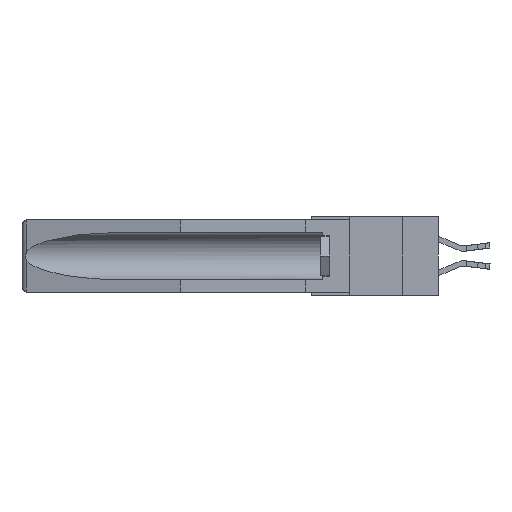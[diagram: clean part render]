
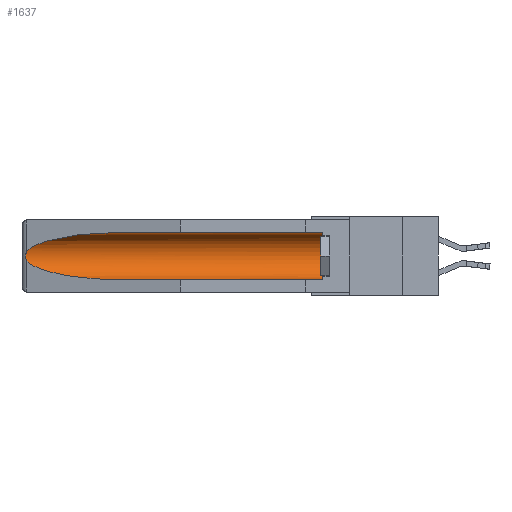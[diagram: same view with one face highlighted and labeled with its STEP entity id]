
A CAD part, left-side view. The second image highlights one B-rep face of the part: STEP entity #1637.
In plain terms, the highlighted cylindrical face has radius 2.857 mm (diameter 5.715 mm), a partial arc.
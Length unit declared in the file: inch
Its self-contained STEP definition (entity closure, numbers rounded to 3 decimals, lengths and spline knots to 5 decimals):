
#1419 = CARTESIAN_POINT ( 'NONE',  ( 0.2675, 1.53308, -0.17534 ) ) ;
#1426 = LINE ( 'NONE', #3609, #10726 ) ;
#1553 = CARTESIAN_POINT ( 'NONE',  ( 0.26537, 1.52718, -0.19328 ) ) ;
#1637 = ADVANCED_FACE ( 'NONE', ( #7533 ), #21561, .F. ) ;
#1683 = CARTESIAN_POINT ( 'NONE',  ( 0.21114, 1.30732, -0.059 ) ) ;
#1746 = EDGE_CURVE ( 'NONE', #3639, #2605, #24716, .T. ) ;
#2605 = VERTEX_POINT ( 'NONE', #8621 ) ;
#3057 = CARTESIAN_POINT ( 'NONE',  ( 0.155, -0.30754, -0.1715 ) ) ;
#3138 = DIRECTION ( 'NONE',  ( 0., 0., 1. ) ) ;
#3371 = CARTESIAN_POINT ( 'NONE',  ( 0.26537, 1.52718, -0.14972 ) ) ;
#3412 = CARTESIAN_POINT ( 'NONE',  ( 0.2673, 1.53269, -0.17917 ) ) ;
#3609 = CARTESIAN_POINT ( 'NONE',  ( 0.155, -0.30754, -0.284 ) ) ;
#3639 = VERTEX_POINT ( 'NONE', #21861 ) ;
#3645 = CARTESIAN_POINT ( 'NONE',  ( 0.155, 1.07973, -0.284 ) ) ;
#5535 = DIRECTION ( 'NONE',  ( 0., 1., 0. ) ) ;
#7226 = VERTEX_POINT ( 'NONE', #24868 ) ;
#7533 = FACE_OUTER_BOUND ( 'NONE', #17918, .T. ) ;
#7554 = DIRECTION ( 'NONE',  ( 0., 1., 0. ) ) ;
#7631 = CARTESIAN_POINT ( 'NONE',  ( 0.26537, 1.52718, -0.14972 ) ) ;
#7634 = EDGE_CURVE ( 'NONE', #20573, #3639, #15903, .T. ) ;
#8621 = CARTESIAN_POINT ( 'NONE',  ( 0.155, 1.07973, -0.059 ) ) ;
#9379 = EDGE_CURVE ( 'NONE', #22008, #7226, #23030, .T. ) ;
#9473 = ORIENTED_EDGE ( 'NONE', *, *, #21713, .T. ) ;
#9589 = CARTESIAN_POINT ( 'NONE',  ( 0.155, 0.126, -0.284 ) ) ;
#9754 = ORIENTED_EDGE ( 'NONE', *, *, #9379, .T. ) ;
#10726 = VECTOR ( 'NONE', #7554, 39.37008 ) ;
#11158 = ORIENTED_EDGE ( 'NONE', *, *, #1746, .T. ) ;
#11304 = CARTESIAN_POINT ( 'NONE',  ( 0.26654, 1.53092, -0.15636 ) ) ;
#11393 = VERTEX_POINT ( 'NONE', #3371 ) ;
#11518 = CARTESIAN_POINT ( 'NONE',  ( 0.155, -0.30754, -0.059 ) ) ;
#12399 = DIRECTION ( 'NONE',  ( 0., 0., 1. ) ) ;
#12753 = EDGE_CURVE ( 'NONE', #20573, #7226, #1426, .T. ) ;
#13455 = CARTESIAN_POINT ( 'NONE',  ( 0.2673, 1.5327, -0.16383 ) ) ;
#13699 = EDGE_CURVE ( 'NONE', #2605, #11393, #17578, .T. ) ;
#14165 = CARTESIAN_POINT ( 'NONE',  ( 0.26537, 1.52718, -0.19328 ) ) ;
#14241 = CARTESIAN_POINT ( 'NONE',  ( 0.155, 0.126, -0.1715 ) ) ;
#15210 = CARTESIAN_POINT ( 'NONE',  ( 0.155, 1.07973, -0.059 ) ) ;
#15285 = CARTESIAN_POINT ( 'NONE',  ( 0.26597, 1.52961, -0.15275 ) ) ;
#15370 = CARTESIAN_POINT ( 'NONE',  ( 0.26537, 1.52718, -0.14972 ) ) ;
#15903 = CIRCLE ( 'NONE', #24970, 0.1125 ) ;
#17293 = CARTESIAN_POINT ( 'NONE',  ( 0.26537, 1.52718, -0.19328 ) ) ;
#17344 = CARTESIAN_POINT ( 'NONE',  ( 0.21114, 1.30732, -0.284 ) ) ;
#17375 = CARTESIAN_POINT ( 'NONE',  ( 0.2675, 1.53308, -0.16763 ) ) ;
#17578 =( BOUNDED_CURVE ( )  B_SPLINE_CURVE ( 3, ( #15210, #1683, #23603, #7631 ),
 .UNSPECIFIED., .F., .T. ) 
 B_SPLINE_CURVE_WITH_KNOTS ( ( 4, 4 ),
 ( 4.71239, 6.08839 ),
 .UNSPECIFIED. ) 
 CURVE ( )  GEOMETRIC_REPRESENTATION_ITEM ( )  RATIONAL_B_SPLINE_CURVE ( ( 1., 0.848, 0.848, 1. ) ) 
 REPRESENTATION_ITEM ( '' )  );
#17918 = EDGE_LOOP ( 'NONE', ( #19096, #9473, #9754, #24249, #18163, #11158 ) ) ;
#18163 = ORIENTED_EDGE ( 'NONE', *, *, #7634, .T. ) ;
#19096 = ORIENTED_EDGE ( 'NONE', *, *, #13699, .T. ) ;
#19286 = CARTESIAN_POINT ( 'NONE',  ( 0.26655, 1.53094, -0.18657 ) ) ;
#19682 = VECTOR ( 'NONE', #5535, 39.37008 ) ;
#20573 = VERTEX_POINT ( 'NONE', #9589 ) ;
#20808 = B_SPLINE_CURVE_WITH_KNOTS ( 'NONE', 3,
 ( #15370, #15285, #11304, #13455, #17375, #1419, #3412, #19286, #21478, #17293 ),
 .UNSPECIFIED., .F., .F.,
 ( 4, 2, 2, 2, 4 ),
 ( 0., 0.00029, 0.00058, 0.00087, 0.00117 ),
 .UNSPECIFIED. ) ;
#21478 = CARTESIAN_POINT ( 'NONE',  ( 0.26597, 1.5296, -0.19026 ) ) ;
#21561 = CYLINDRICAL_SURFACE ( 'NONE', #23545, 0.1125 ) ;
#21713 = EDGE_CURVE ( 'NONE', #11393, #22008, #20808, .T. ) ;
#21861 = CARTESIAN_POINT ( 'NONE',  ( 0.155, 0.126, -0.059 ) ) ;
#22008 = VERTEX_POINT ( 'NONE', #14165 ) ;
#22167 = DIRECTION ( 'NONE',  ( 0., -1., 0. ) ) ;
#23030 =( BOUNDED_CURVE ( )  B_SPLINE_CURVE ( 3, ( #1553, #25505, #17344, #3645 ),
 .UNSPECIFIED., .F., .F. ) 
 B_SPLINE_CURVE_WITH_KNOTS ( ( 4, 4 ),
 ( 0.1948, 1.5708 ),
 .UNSPECIFIED. ) 
 CURVE ( )  GEOMETRIC_REPRESENTATION_ITEM ( )  RATIONAL_B_SPLINE_CURVE ( ( 1., 0.848, 0.848, 1. ) ) 
 REPRESENTATION_ITEM ( '' )  );
#23545 = AXIS2_PLACEMENT_3D ( 'NONE', #3057, #24976, #3138 ) ;
#23603 = CARTESIAN_POINT ( 'NONE',  ( 0.25451, 1.48313, -0.09465 ) ) ;
#24249 = ORIENTED_EDGE ( 'NONE', *, *, #12753, .F. ) ;
#24716 = LINE ( 'NONE', #11518, #19682 ) ;
#24868 = CARTESIAN_POINT ( 'NONE',  ( 0.155, 1.07973, -0.284 ) ) ;
#24970 = AXIS2_PLACEMENT_3D ( 'NONE', #14241, #22167, #12399 ) ;
#24976 = DIRECTION ( 'NONE',  ( 0., 1., 0. ) ) ;
#25505 = CARTESIAN_POINT ( 'NONE',  ( 0.25451, 1.48313, -0.24835 ) ) ;
